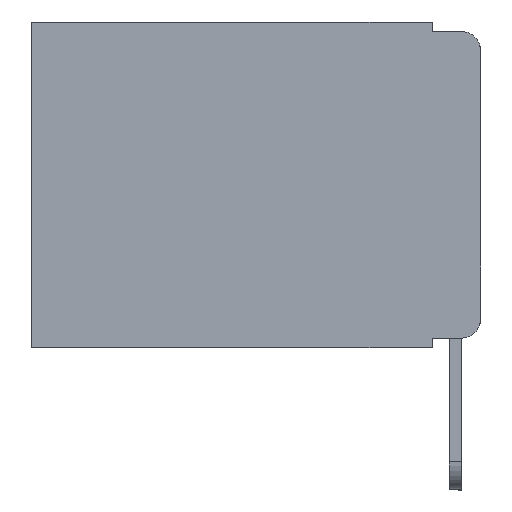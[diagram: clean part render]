
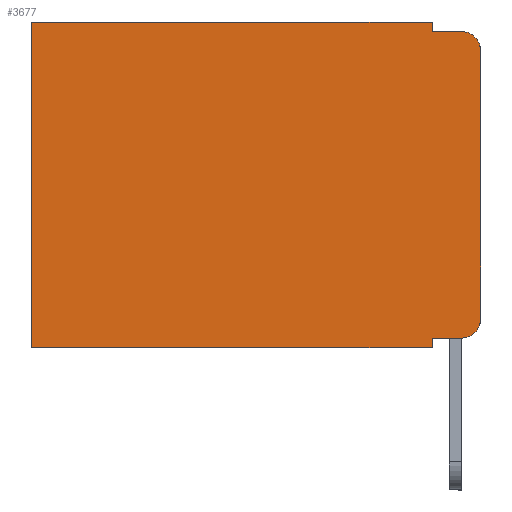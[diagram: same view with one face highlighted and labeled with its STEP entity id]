
A CAD part, left-side view. The second image highlights one B-rep face of the part: STEP entity #3677.
In plain terms, the highlighted planar face has unit normal (-1, 0, 0).
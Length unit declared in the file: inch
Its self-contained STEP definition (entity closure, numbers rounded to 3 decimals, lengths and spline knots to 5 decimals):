
#36 = DIRECTION ( 'NONE',  ( 0., -1., 0. ) ) ;
#57 = DIRECTION ( 'NONE',  ( 0., 0., -1. ) ) ;
#145 = CARTESIAN_POINT ( 'NONE',  ( 0.298, 0., -0.343 ) ) ;
#388 = CARTESIAN_POINT ( 'NONE',  ( 0.298, 0.051, 0. ) ) ;
#399 = LINE ( 'NONE', #2248, #22528 ) ;
#638 = EDGE_CURVE ( 'NONE', #11038, #17831, #3648, .T. ) ;
#1298 = CARTESIAN_POINT ( 'NONE',  ( 0.298, 0.051, -0.01 ) ) ;
#1420 = CARTESIAN_POINT ( 'NONE',  ( 0.298, 0.051, 0. ) ) ;
#1469 = ORIENTED_EDGE ( 'NONE', *, *, #20382, .F. ) ;
#1484 = LINE ( 'NONE', #12321, #7746 ) ;
#1665 = VERTEX_POINT ( 'NONE', #21936 ) ;
#2248 = CARTESIAN_POINT ( 'NONE',  ( 0.298, 0.473, 0. ) ) ;
#2407 = ORIENTED_EDGE ( 'NONE', *, *, #16040, .F. ) ;
#3104 = ORIENTED_EDGE ( 'NONE', *, *, #19215, .T. ) ;
#3648 = LINE ( 'NONE', #4112, #11597 ) ;
#3660 = VERTEX_POINT ( 'NONE', #388 ) ;
#3677 = ADVANCED_FACE ( 'NONE', ( #4093 ), #9251, .F. ) ;
#3939 = LINE ( 'NONE', #14518, #12279 ) ;
#4093 = FACE_OUTER_BOUND ( 'NONE', #19313, .T. ) ;
#4112 = CARTESIAN_POINT ( 'NONE',  ( 0.298, 0.051, -0.333 ) ) ;
#4603 = CIRCLE ( 'NONE', #11571, 0.02 ) ;
#5186 = EDGE_CURVE ( 'NONE', #14152, #6066, #399, .T. ) ;
#5326 = ORIENTED_EDGE ( 'NONE', *, *, #8161, .T. ) ;
#5778 = VECTOR ( 'NONE', #19494, 39.37008 ) ;
#5971 = VECTOR ( 'NONE', #6069, 39.37008 ) ;
#6056 = DIRECTION ( 'NONE',  ( -1., 0., 0. ) ) ;
#6066 = VERTEX_POINT ( 'NONE', #7826 ) ;
#6069 = DIRECTION ( 'NONE',  ( 0., 0., -1. ) ) ;
#6284 = AXIS2_PLACEMENT_3D ( 'NONE', #21808, #6056, #13073 ) ;
#6569 = EDGE_CURVE ( 'NONE', #1665, #15284, #12982, .T. ) ;
#6606 = AXIS2_PLACEMENT_3D ( 'NONE', #7540, #21552, #12823 ) ;
#7014 = DIRECTION ( 'NONE',  ( 0., 0., -1. ) ) ;
#7287 = CARTESIAN_POINT ( 'NONE',  ( 0.298, 0.051, -0.333 ) ) ;
#7540 = CARTESIAN_POINT ( 'NONE',  ( 0.298, 0., 0. ) ) ;
#7746 = VECTOR ( 'NONE', #7014, 39.37008 ) ;
#7826 = CARTESIAN_POINT ( 'NONE',  ( 0.298, 0.473, -0.343 ) ) ;
#8161 = EDGE_CURVE ( 'NONE', #17831, #15284, #4603, .T. ) ;
#8755 = VERTEX_POINT ( 'NONE', #10723 ) ;
#9095 = CARTESIAN_POINT ( 'NONE',  ( 0.298, 0.02, -0.333 ) ) ;
#9251 = PLANE ( 'NONE',  #6606 ) ;
#9834 = EDGE_CURVE ( 'NONE', #8755, #6066, #22698, .T. ) ;
#9838 = ORIENTED_EDGE ( 'NONE', *, *, #15424, .T. ) ;
#10396 = LINE ( 'NONE', #1420, #22640 ) ;
#10723 = CARTESIAN_POINT ( 'NONE',  ( 0.298, 0.051, -0.343 ) ) ;
#11038 = VERTEX_POINT ( 'NONE', #7287 ) ;
#11054 = DIRECTION ( 'NONE',  ( 0., 1., 0. ) ) ;
#11571 = AXIS2_PLACEMENT_3D ( 'NONE', #12273, #15601, #57 ) ;
#11597 = VECTOR ( 'NONE', #17795, 39.37008 ) ;
#12273 = CARTESIAN_POINT ( 'NONE',  ( 0.298, 0.02, -0.313 ) ) ;
#12279 = VECTOR ( 'NONE', #11054, 39.37008 ) ;
#12321 = CARTESIAN_POINT ( 'NONE',  ( 0.298, 0.051, 0. ) ) ;
#12823 = DIRECTION ( 'NONE',  ( 0., 0., -1. ) ) ;
#12860 = ORIENTED_EDGE ( 'NONE', *, *, #6569, .F. ) ;
#12982 = LINE ( 'NONE', #18164, #5971 ) ;
#13073 = DIRECTION ( 'NONE',  ( 0., 0., -1. ) ) ;
#14152 = VERTEX_POINT ( 'NONE', #22220 ) ;
#14214 = DIRECTION ( 'NONE',  ( 0., 0., -1. ) ) ;
#14242 = ORIENTED_EDGE ( 'NONE', *, *, #9834, .F. ) ;
#14351 = VERTEX_POINT ( 'NONE', #17168 ) ;
#14518 = CARTESIAN_POINT ( 'NONE',  ( 0.298, 0., 0. ) ) ;
#14739 = EDGE_CURVE ( 'NONE', #11038, #8755, #1484, .T. ) ;
#15284 = VERTEX_POINT ( 'NONE', #21245 ) ;
#15424 = EDGE_CURVE ( 'NONE', #1665, #16677, #16222, .T. ) ;
#15456 = ORIENTED_EDGE ( 'NONE', *, *, #5186, .T. ) ;
#15601 = DIRECTION ( 'NONE',  ( -1., 0., 0. ) ) ;
#16040 = EDGE_CURVE ( 'NONE', #14351, #16677, #22584, .T. ) ;
#16222 = CIRCLE ( 'NONE', #6284, 0.02 ) ;
#16677 = VERTEX_POINT ( 'NONE', #18607 ) ;
#17168 = CARTESIAN_POINT ( 'NONE',  ( 0.298, 0.051, -0.01 ) ) ;
#17430 = DIRECTION ( 'NONE',  ( 0., 0., -1. ) ) ;
#17795 = DIRECTION ( 'NONE',  ( 0., -1., 0. ) ) ;
#17831 = VERTEX_POINT ( 'NONE', #9095 ) ;
#18164 = CARTESIAN_POINT ( 'NONE',  ( 0.298, 0., 0. ) ) ;
#18607 = CARTESIAN_POINT ( 'NONE',  ( 0.298, 0.02, -0.01 ) ) ;
#19215 = EDGE_CURVE ( 'NONE', #3660, #14152, #3939, .T. ) ;
#19313 = EDGE_LOOP ( 'NONE', ( #12860, #9838, #2407, #1469, #3104, #15456, #14242, #20752, #20784, #5326 ) ) ;
#19494 = DIRECTION ( 'NONE',  ( 0., 1., 0. ) ) ;
#20382 = EDGE_CURVE ( 'NONE', #3660, #14351, #10396, .T. ) ;
#20752 = ORIENTED_EDGE ( 'NONE', *, *, #14739, .F. ) ;
#20784 = ORIENTED_EDGE ( 'NONE', *, *, #638, .T. ) ;
#21245 = CARTESIAN_POINT ( 'NONE',  ( 0.298, 0., -0.313 ) ) ;
#21552 = DIRECTION ( 'NONE',  ( 1., 0., 0. ) ) ;
#21808 = CARTESIAN_POINT ( 'NONE',  ( 0.298, 0.02, -0.03 ) ) ;
#21936 = CARTESIAN_POINT ( 'NONE',  ( 0.298, 0., -0.03 ) ) ;
#22220 = CARTESIAN_POINT ( 'NONE',  ( 0.298, 0.473, 0. ) ) ;
#22467 = VECTOR ( 'NONE', #36, 39.37008 ) ;
#22528 = VECTOR ( 'NONE', #14214, 39.37008 ) ;
#22584 = LINE ( 'NONE', #1298, #22467 ) ;
#22640 = VECTOR ( 'NONE', #17430, 39.37008 ) ;
#22698 = LINE ( 'NONE', #145, #5778 ) ;
